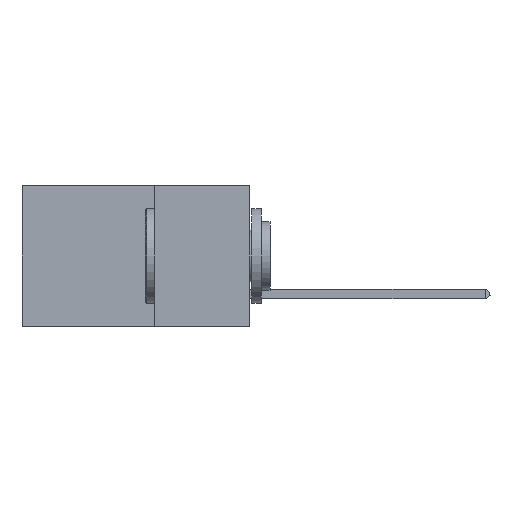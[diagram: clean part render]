
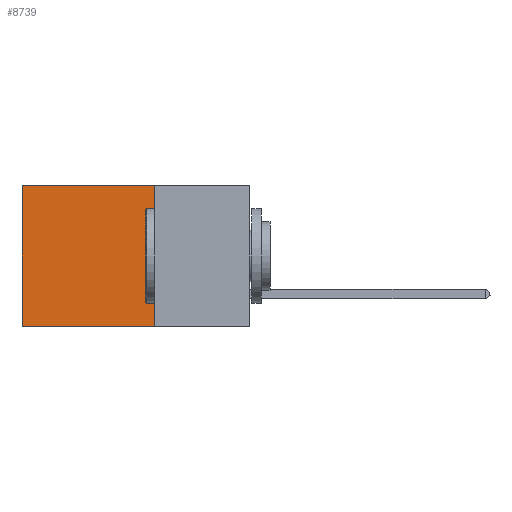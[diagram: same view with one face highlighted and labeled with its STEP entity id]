
A CAD part, left-side view. The second image highlights one B-rep face of the part: STEP entity #8739.
In plain terms, the highlighted planar face has unit normal (-1, 0, 0).
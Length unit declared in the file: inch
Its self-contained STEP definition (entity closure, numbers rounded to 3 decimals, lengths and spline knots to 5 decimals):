
#819 = DIRECTION ( 'NONE',  ( 0., 0., -1. ) ) ;
#899 = EDGE_CURVE ( 'NONE', #5631, #6142, #10225, .T. ) ;
#2229 = EDGE_CURVE ( 'NONE', #2352, #6142, #12278, .T. ) ;
#2352 = VERTEX_POINT ( 'NONE', #14917 ) ;
#3051 = VECTOR ( 'NONE', #13346, 39.37008 ) ;
#3419 = DIRECTION ( 'NONE',  ( 1., 0., 0. ) ) ;
#3552 = CARTESIAN_POINT ( 'NONE',  ( 0.2875, 0.25, 0. ) ) ;
#3586 = DIRECTION ( 'NONE',  ( 0., 0., -1. ) ) ;
#3825 = ORIENTED_EDGE ( 'NONE', *, *, #12741, .T. ) ;
#3890 = ORIENTED_EDGE ( 'NONE', *, *, #899, .F. ) ;
#4632 = LINE ( 'NONE', #6147, #7442 ) ;
#4711 = LINE ( 'NONE', #7048, #10882 ) ;
#5002 = EDGE_LOOP ( 'NONE', ( #9713, #3890, #15469, #3825 ) ) ;
#5631 = VERTEX_POINT ( 'NONE', #7065 ) ;
#6142 = VERTEX_POINT ( 'NONE', #9267 ) ;
#6147 = CARTESIAN_POINT ( 'NONE',  ( 0.2875, 0.25, 0. ) ) ;
#7048 = CARTESIAN_POINT ( 'NONE',  ( 0.2875, 0.25, 0. ) ) ;
#7065 = CARTESIAN_POINT ( 'NONE',  ( 0.2875, 0.25, -0.37 ) ) ;
#7442 = VECTOR ( 'NONE', #13275, 39.37008 ) ;
#8660 = CARTESIAN_POINT ( 'NONE',  ( 0.2875, 0.6, 0. ) ) ;
#8739 = ADVANCED_FACE ( 'NONE', ( #9266 ), #13162, .F. ) ;
#9266 = FACE_OUTER_BOUND ( 'NONE', #5002, .T. ) ;
#9267 = CARTESIAN_POINT ( 'NONE',  ( 0.2875, 0.6, -0.37 ) ) ;
#9531 = DIRECTION ( 'NONE',  ( 0., 1., 0. ) ) ;
#9566 = CARTESIAN_POINT ( 'NONE',  ( 0.2875, 0.25, 0. ) ) ;
#9636 = AXIS2_PLACEMENT_3D ( 'NONE', #9566, #3419, #3586 ) ;
#9713 = ORIENTED_EDGE ( 'NONE', *, *, #2229, .T. ) ;
#10225 = LINE ( 'NONE', #15543, #12709 ) ;
#10882 = VECTOR ( 'NONE', #819, 39.37008 ) ;
#12278 = LINE ( 'NONE', #8660, #3051 ) ;
#12587 = VERTEX_POINT ( 'NONE', #3552 ) ;
#12709 = VECTOR ( 'NONE', #9531, 39.37008 ) ;
#12741 = EDGE_CURVE ( 'NONE', #12587, #2352, #4632, .T. ) ;
#13162 = PLANE ( 'NONE',  #9636 ) ;
#13275 = DIRECTION ( 'NONE',  ( 0., 1., 0. ) ) ;
#13346 = DIRECTION ( 'NONE',  ( 0., 0., -1. ) ) ;
#13656 = EDGE_CURVE ( 'NONE', #12587, #5631, #4711, .T. ) ;
#14917 = CARTESIAN_POINT ( 'NONE',  ( 0.2875, 0.6, 0. ) ) ;
#15469 = ORIENTED_EDGE ( 'NONE', *, *, #13656, .F. ) ;
#15543 = CARTESIAN_POINT ( 'NONE',  ( 0.2875, 0.25, -0.37 ) ) ;
